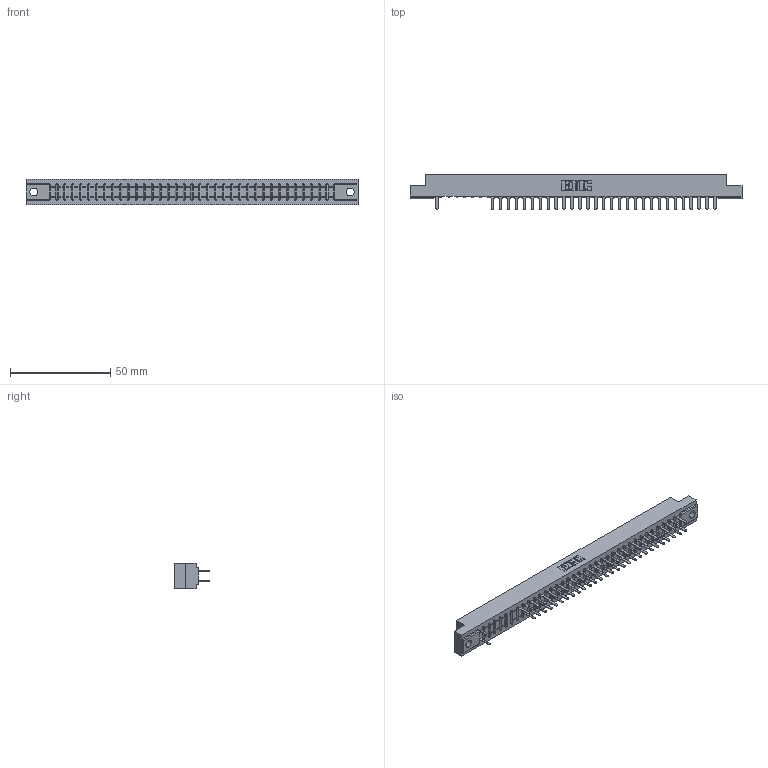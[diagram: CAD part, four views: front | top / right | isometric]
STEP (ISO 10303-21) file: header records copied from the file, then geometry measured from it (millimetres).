
FILE_DESCRIPTION (( 'STEP AP203' ), '1' );
FILE_NAME ('307-072-520-204.STEP', '2018-08-06T13:41:44', ( '' ), ( '' ), 'SwSTEP 2.0', 'SolidWorks 2016', '' );
FILE_SCHEMA (( 'CONFIG_CONTROL_DESIGN' ));
Length unit declared in the file: inch
Products named in the file (3): 307 Part_.156 Dia Mounting Holes; 307-290-001_520; 307-072-520-204
Assembly tree (60 placements, depth 2):
  307-072-520-204
    307 Part_.156 Dia Mounting Holes
    307-290-001_520  x59
Bounding box: 165.66 x 17.42 x 12.7 mm (x, y, z)
Volume: 17342.3 mm3; surface area: 19921.2 mm2
Topology: 60 solids, 60 shells, 3013 faces, 8445 edges, 5450 vertices
Faces by surface type: plane 1991, cylinder 948, sphere 74
Entity records: 32724 total; most frequent: CARTESIAN_POINT 5413, ORIENTED_EDGE 5374, DIRECTION 5283, EDGE_CURVE 2687, LINE 2067, VECTOR 2067, VERTEX_POINT 1738, AXIS2_PLACEMENT_3D 1608
